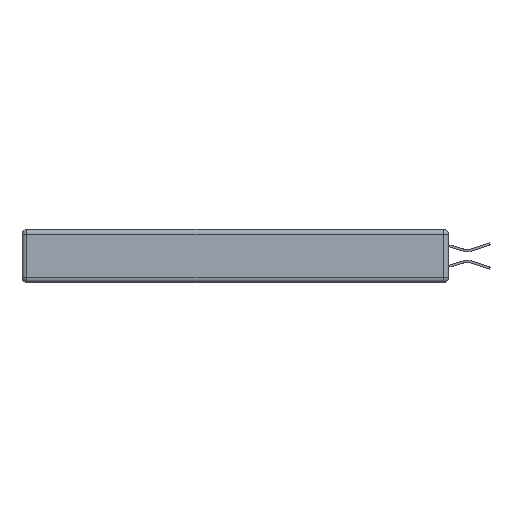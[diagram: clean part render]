
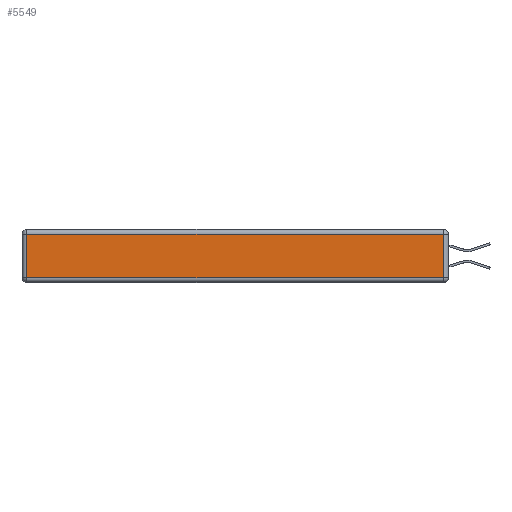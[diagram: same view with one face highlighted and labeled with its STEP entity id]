
A CAD part, left-side view. The second image highlights one B-rep face of the part: STEP entity #5549.
In plain terms, the highlighted planar face has unit normal (-1, 0, 0).
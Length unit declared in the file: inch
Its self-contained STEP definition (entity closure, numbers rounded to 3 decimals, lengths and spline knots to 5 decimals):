
#654 = DIRECTION ( 'NONE',  ( 0., 1., 0. ) ) ;
#655 = VECTOR ( 'NONE', #13807, 39.37008 ) ;
#1092 = CARTESIAN_POINT ( 'NONE',  ( 0., 0.03, -0.343 ) ) ;
#1584 = DIRECTION ( 'NONE',  ( 0., -1., 0. ) ) ;
#1677 = LINE ( 'NONE', #1092, #6255 ) ;
#2551 = DIRECTION ( 'NONE',  ( 0., 0., 1. ) ) ;
#2901 = VERTEX_POINT ( 'NONE', #2908 ) ;
#2908 = CARTESIAN_POINT ( 'NONE',  ( 0., 0.03, -0.03 ) ) ;
#3334 = FACE_OUTER_BOUND ( 'NONE', #12831, .T. ) ;
#3554 = ORIENTED_EDGE ( 'NONE', *, *, #3713, .T. ) ;
#3713 = EDGE_CURVE ( 'NONE', #16630, #10653, #10468, .T. ) ;
#4126 = CARTESIAN_POINT ( 'NONE',  ( 0., 0., -0.313 ) ) ;
#4608 = CARTESIAN_POINT ( 'NONE',  ( 0., 2.75, -0.03 ) ) ;
#5112 = DIRECTION ( 'NONE',  ( -1., 0., 0. ) ) ;
#5549 = ADVANCED_FACE ( 'NONE', ( #3334 ), #10548, .T. ) ;
#5676 = EDGE_CURVE ( 'NONE', #10653, #2901, #1677, .T. ) ;
#6252 = EDGE_CURVE ( 'NONE', #2901, #13777, #13512, .T. ) ;
#6255 = VECTOR ( 'NONE', #17131, 39.37008 ) ;
#6515 = VECTOR ( 'NONE', #1584, 39.37008 ) ;
#6853 = EDGE_CURVE ( 'NONE', #13777, #16630, #10841, .T. ) ;
#7134 = CARTESIAN_POINT ( 'NONE',  ( 0., 2.72, -0.313 ) ) ;
#7688 = CARTESIAN_POINT ( 'NONE',  ( 0., 0., -0.343 ) ) ;
#7874 = ORIENTED_EDGE ( 'NONE', *, *, #6853, .T. ) ;
#9080 = CARTESIAN_POINT ( 'NONE',  ( 0., 0.03, -0.313 ) ) ;
#9573 = VECTOR ( 'NONE', #654, 39.37008 ) ;
#9893 = CARTESIAN_POINT ( 'NONE',  ( 0., 2.72, -0.343 ) ) ;
#10468 = LINE ( 'NONE', #4126, #6515 ) ;
#10548 = PLANE ( 'NONE',  #12110 ) ;
#10653 = VERTEX_POINT ( 'NONE', #9080 ) ;
#10841 = LINE ( 'NONE', #9893, #655 ) ;
#12110 = AXIS2_PLACEMENT_3D ( 'NONE', #7688, #5112, #2551 ) ;
#12831 = EDGE_LOOP ( 'NONE', ( #3554, #17150, #15512, #7874 ) ) ;
#13149 = CARTESIAN_POINT ( 'NONE',  ( 0., 2.72, -0.03 ) ) ;
#13512 = LINE ( 'NONE', #4608, #9573 ) ;
#13777 = VERTEX_POINT ( 'NONE', #13149 ) ;
#13807 = DIRECTION ( 'NONE',  ( 0., 0., -1. ) ) ;
#15512 = ORIENTED_EDGE ( 'NONE', *, *, #6252, .T. ) ;
#16630 = VERTEX_POINT ( 'NONE', #7134 ) ;
#17131 = DIRECTION ( 'NONE',  ( 0., 0., 1. ) ) ;
#17150 = ORIENTED_EDGE ( 'NONE', *, *, #5676, .T. ) ;
